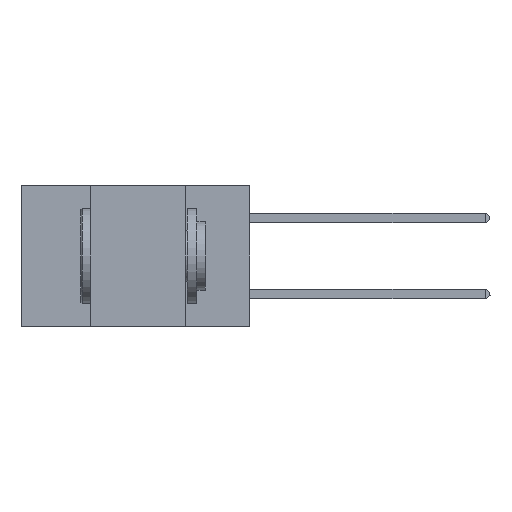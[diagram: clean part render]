
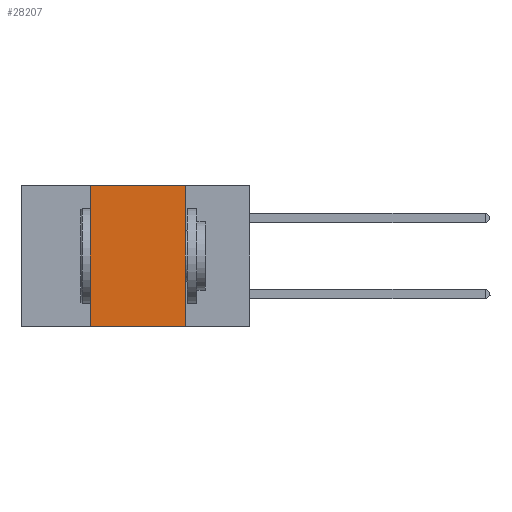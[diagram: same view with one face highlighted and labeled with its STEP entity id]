
A CAD part, left-side view. The second image highlights one B-rep face of the part: STEP entity #28207.
In plain terms, the highlighted planar face has unit normal (-1, 0, 0).
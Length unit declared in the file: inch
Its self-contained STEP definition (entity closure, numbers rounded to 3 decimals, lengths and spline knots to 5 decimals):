
#1561 = VECTOR ( 'NONE', #25955, 39.37008 ) ;
#2141 = EDGE_CURVE ( 'NONE', #37188, #36420, #6539, .T. ) ;
#3297 = VECTOR ( 'NONE', #11387, 39.37008 ) ;
#3683 = ORIENTED_EDGE ( 'NONE', *, *, #2141, .F. ) ;
#4473 = ORIENTED_EDGE ( 'NONE', *, *, #38700, .T. ) ;
#4504 = ORIENTED_EDGE ( 'NONE', *, *, #36643, .F. ) ;
#5020 = DIRECTION ( 'NONE',  ( 0., 0., -1. ) ) ;
#5690 = CARTESIAN_POINT ( 'NONE',  ( 0., 0.17, 0. ) ) ;
#6539 = LINE ( 'NONE', #5690, #26979 ) ;
#6789 = AXIS2_PLACEMENT_3D ( 'NONE', #30316, #17691, #5020 ) ;
#7187 = CARTESIAN_POINT ( 'NONE',  ( 0., 0.42, 0. ) ) ;
#11387 = DIRECTION ( 'NONE',  ( 0., -1., 0. ) ) ;
#11529 = EDGE_CURVE ( 'NONE', #18034, #37188, #12610, .T. ) ;
#12610 = LINE ( 'NONE', #18423, #38392 ) ;
#14825 = PLANE ( 'NONE',  #6789 ) ;
#15532 = LINE ( 'NONE', #18082, #3297 ) ;
#17691 = DIRECTION ( 'NONE',  ( 1., 0., 0. ) ) ;
#18034 = VERTEX_POINT ( 'NONE', #20512 ) ;
#18082 = CARTESIAN_POINT ( 'NONE',  ( 0., 0.6, -0.37 ) ) ;
#18423 = CARTESIAN_POINT ( 'NONE',  ( 0., 0.6, 0. ) ) ;
#18816 = DIRECTION ( 'NONE',  ( 0., -1., 0. ) ) ;
#19419 = ORIENTED_EDGE ( 'NONE', *, *, #11529, .F. ) ;
#20512 = CARTESIAN_POINT ( 'NONE',  ( 0., 0.42, 0. ) ) ;
#25955 = DIRECTION ( 'NONE',  ( 0., 0., 1. ) ) ;
#26979 = VECTOR ( 'NONE', #29627, 39.37008 ) ;
#28207 = ADVANCED_FACE ( 'NONE', ( #38916 ), #14825, .F. ) ;
#28757 = EDGE_LOOP ( 'NONE', ( #3683, #19419, #4504, #4473 ) ) ;
#29627 = DIRECTION ( 'NONE',  ( 0., 0., -1. ) ) ;
#30316 = CARTESIAN_POINT ( 'NONE',  ( 0., 0.6, 0. ) ) ;
#30895 = CARTESIAN_POINT ( 'NONE',  ( 0., 0.42, -0.37 ) ) ;
#31558 = CARTESIAN_POINT ( 'NONE',  ( 0., 0.17, -0.37 ) ) ;
#31647 = CARTESIAN_POINT ( 'NONE',  ( 0., 0.17, 0. ) ) ;
#34664 = LINE ( 'NONE', #7187, #1561 ) ;
#35272 = VERTEX_POINT ( 'NONE', #30895 ) ;
#36420 = VERTEX_POINT ( 'NONE', #31558 ) ;
#36643 = EDGE_CURVE ( 'NONE', #35272, #18034, #34664, .T. ) ;
#37188 = VERTEX_POINT ( 'NONE', #31647 ) ;
#38392 = VECTOR ( 'NONE', #18816, 39.37008 ) ;
#38700 = EDGE_CURVE ( 'NONE', #35272, #36420, #15532, .T. ) ;
#38916 = FACE_OUTER_BOUND ( 'NONE', #28757, .T. ) ;
